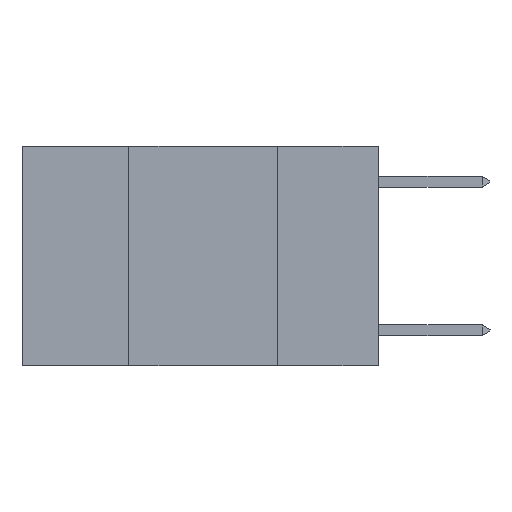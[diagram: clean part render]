
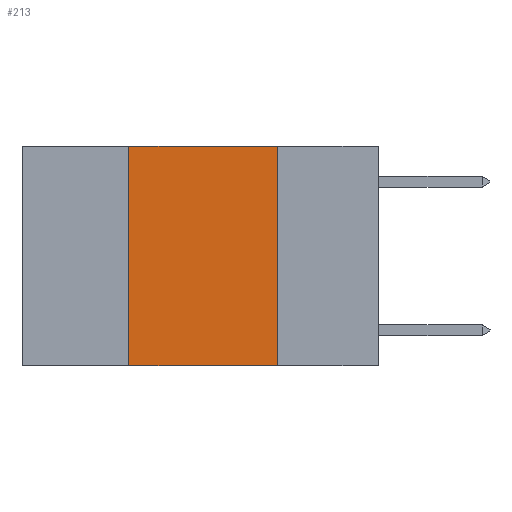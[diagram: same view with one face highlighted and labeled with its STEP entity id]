
A CAD part, left-side view. The second image highlights one B-rep face of the part: STEP entity #213.
In plain terms, the highlighted planar face has unit normal (-1, 0, 0).
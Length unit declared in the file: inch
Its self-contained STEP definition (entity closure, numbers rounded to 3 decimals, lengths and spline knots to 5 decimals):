
#213 = ADVANCED_FACE ( 'NONE', ( #5695 ), #7410, .F. ) ;
#672 = EDGE_LOOP ( 'NONE', ( #8440, #8085, #9514, #1467 ) ) ;
#1031 = CARTESIAN_POINT ( 'NONE',  ( 0., 0.6, 0. ) ) ;
#1450 = DIRECTION ( 'NONE',  ( 0., -1., 0. ) ) ;
#1467 = ORIENTED_EDGE ( 'NONE', *, *, #8538, .T. ) ;
#1601 = VERTEX_POINT ( 'NONE', #2545 ) ;
#1794 = VERTEX_POINT ( 'NONE', #3096 ) ;
#2486 = CARTESIAN_POINT ( 'NONE',  ( 0., 0.17, 0. ) ) ;
#2545 = CARTESIAN_POINT ( 'NONE',  ( 0., 0.42, 0. ) ) ;
#3096 = CARTESIAN_POINT ( 'NONE',  ( 0., 0.42, -0.37 ) ) ;
#3269 = VECTOR ( 'NONE', #6234, 39.37008 ) ;
#3821 = EDGE_CURVE ( 'NONE', #1794, #1601, #7050, .T. ) ;
#3940 = AXIS2_PLACEMENT_3D ( 'NONE', #1031, #4356, #6220 ) ;
#4038 = CARTESIAN_POINT ( 'NONE',  ( 0., 0.17, 0. ) ) ;
#4170 = LINE ( 'NONE', #4999, #9525 ) ;
#4356 = DIRECTION ( 'NONE',  ( 1., 0., 0. ) ) ;
#4471 = CARTESIAN_POINT ( 'NONE',  ( 0., 0.17, -0.37 ) ) ;
#4842 = EDGE_CURVE ( 'NONE', #1601, #7092, #4170, .T. ) ;
#4999 = CARTESIAN_POINT ( 'NONE',  ( 0., 0.6, 0. ) ) ;
#5380 = LINE ( 'NONE', #4038, #8659 ) ;
#5431 = EDGE_CURVE ( 'NONE', #7092, #9445, #5380, .T. ) ;
#5681 = DIRECTION ( 'NONE',  ( 0., -1., 0. ) ) ;
#5695 = FACE_OUTER_BOUND ( 'NONE', #672, .T. ) ;
#5779 = CARTESIAN_POINT ( 'NONE',  ( 0., 0.6, -0.37 ) ) ;
#6220 = DIRECTION ( 'NONE',  ( 0., 0., -1. ) ) ;
#6234 = DIRECTION ( 'NONE',  ( 0., 0., 1. ) ) ;
#6870 = DIRECTION ( 'NONE',  ( 0., 0., -1. ) ) ;
#6925 = CARTESIAN_POINT ( 'NONE',  ( 0., 0.42, 0. ) ) ;
#7050 = LINE ( 'NONE', #6925, #3269 ) ;
#7092 = VERTEX_POINT ( 'NONE', #2486 ) ;
#7410 = PLANE ( 'NONE',  #3940 ) ;
#7822 = LINE ( 'NONE', #5779, #9465 ) ;
#8085 = ORIENTED_EDGE ( 'NONE', *, *, #4842, .F. ) ;
#8440 = ORIENTED_EDGE ( 'NONE', *, *, #5431, .F. ) ;
#8538 = EDGE_CURVE ( 'NONE', #1794, #9445, #7822, .T. ) ;
#8659 = VECTOR ( 'NONE', #6870, 39.37008 ) ;
#9445 = VERTEX_POINT ( 'NONE', #4471 ) ;
#9465 = VECTOR ( 'NONE', #1450, 39.37008 ) ;
#9514 = ORIENTED_EDGE ( 'NONE', *, *, #3821, .F. ) ;
#9525 = VECTOR ( 'NONE', #5681, 39.37008 ) ;
